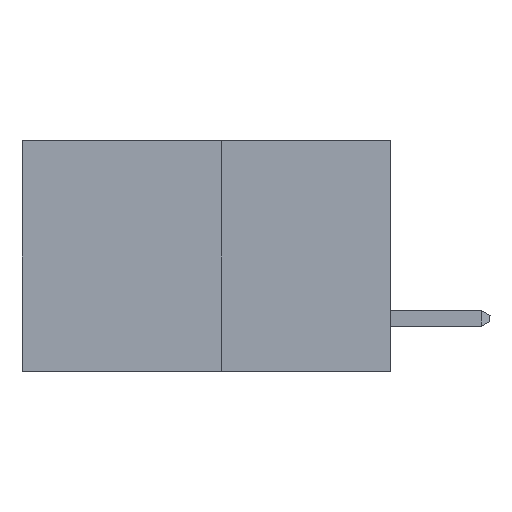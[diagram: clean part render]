
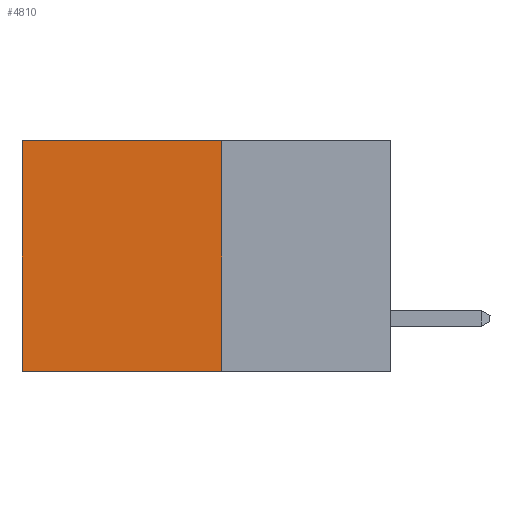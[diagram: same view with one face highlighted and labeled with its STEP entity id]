
A CAD part, left-side view. The second image highlights one B-rep face of the part: STEP entity #4810.
In plain terms, the highlighted planar face has unit normal (-1, 0, 0).
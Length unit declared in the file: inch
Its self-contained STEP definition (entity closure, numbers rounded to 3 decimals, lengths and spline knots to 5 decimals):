
#112 = VECTOR ( 'NONE', #10552, 39.37008 ) ;
#391 = DIRECTION ( 'NONE',  ( 0., 0., -1. ) ) ;
#427 = DIRECTION ( 'NONE',  ( 0., 1., 0. ) ) ;
#618 = LINE ( 'NONE', #7628, #9328 ) ;
#1446 = VERTEX_POINT ( 'NONE', #5433 ) ;
#1479 = DIRECTION ( 'NONE',  ( 0., 1., 0. ) ) ;
#2505 = AXIS2_PLACEMENT_3D ( 'NONE', #7114, #7051, #7325 ) ;
#2518 = LINE ( 'NONE', #10467, #112 ) ;
#2660 = VERTEX_POINT ( 'NONE', #4114 ) ;
#3164 = VERTEX_POINT ( 'NONE', #9521 ) ;
#3902 = LINE ( 'NONE', #10769, #5984 ) ;
#4114 = CARTESIAN_POINT ( 'NONE',  ( 0.277, 0.27, 0. ) ) ;
#4193 = VECTOR ( 'NONE', #391, 39.37008 ) ;
#4586 = ORIENTED_EDGE ( 'NONE', *, *, #5770, .F. ) ;
#4810 = ADVANCED_FACE ( 'NONE', ( #9794 ), #10115, .F. ) ;
#4851 = ORIENTED_EDGE ( 'NONE', *, *, #10401, .F. ) ;
#4960 = ORIENTED_EDGE ( 'NONE', *, *, #9846, .T. ) ;
#4988 = ORIENTED_EDGE ( 'NONE', *, *, #10373, .T. ) ;
#5178 = EDGE_LOOP ( 'NONE', ( #4988, #4851, #4586, #4960 ) ) ;
#5433 = CARTESIAN_POINT ( 'NONE',  ( 0.277, 0.59, 0. ) ) ;
#5770 = EDGE_CURVE ( 'NONE', #2660, #3164, #2518, .T. ) ;
#5812 = CARTESIAN_POINT ( 'NONE',  ( 0.277, 0.59, -0.37 ) ) ;
#5891 = CARTESIAN_POINT ( 'NONE',  ( 0.277, 0.59, -0.37 ) ) ;
#5984 = VECTOR ( 'NONE', #427, 39.37008 ) ;
#6809 = VERTEX_POINT ( 'NONE', #5891 ) ;
#7051 = DIRECTION ( 'NONE',  ( 1., 0., 0. ) ) ;
#7114 = CARTESIAN_POINT ( 'NONE',  ( 0.277, 0.27, -0.37 ) ) ;
#7325 = DIRECTION ( 'NONE',  ( 0., 0., -1. ) ) ;
#7628 = CARTESIAN_POINT ( 'NONE',  ( 0.277, 0.27, 0. ) ) ;
#9328 = VECTOR ( 'NONE', #1479, 39.37008 ) ;
#9521 = CARTESIAN_POINT ( 'NONE',  ( 0.277, 0.27, -0.37 ) ) ;
#9794 = FACE_OUTER_BOUND ( 'NONE', #5178, .T. ) ;
#9846 = EDGE_CURVE ( 'NONE', #2660, #1446, #618, .T. ) ;
#10115 = PLANE ( 'NONE',  #2505 ) ;
#10373 = EDGE_CURVE ( 'NONE', #1446, #6809, #10621, .T. ) ;
#10401 = EDGE_CURVE ( 'NONE', #3164, #6809, #3902, .T. ) ;
#10467 = CARTESIAN_POINT ( 'NONE',  ( 0.277, 0.27, -0.37 ) ) ;
#10552 = DIRECTION ( 'NONE',  ( 0., 0., -1. ) ) ;
#10621 = LINE ( 'NONE', #5812, #4193 ) ;
#10769 = CARTESIAN_POINT ( 'NONE',  ( 0.277, 0.27, -0.37 ) ) ;
